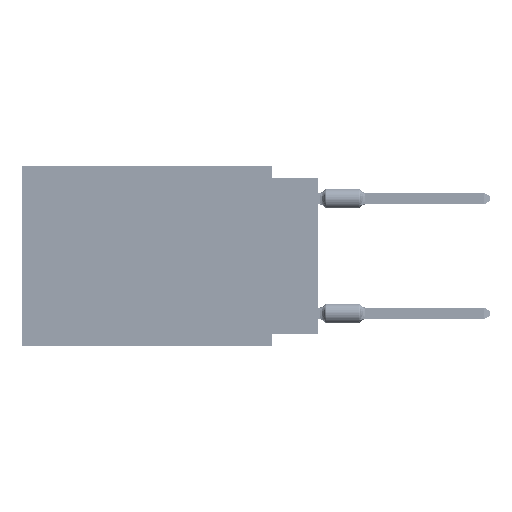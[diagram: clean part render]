
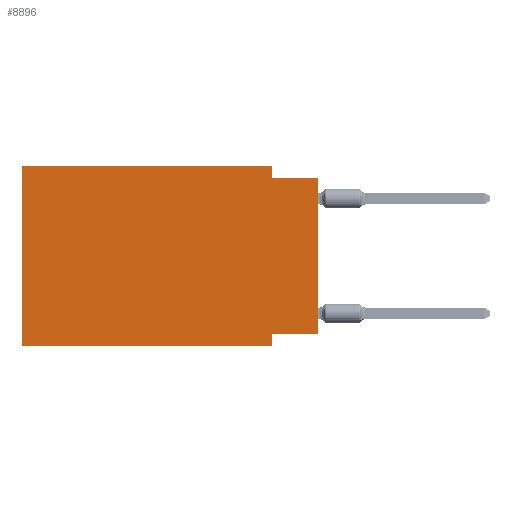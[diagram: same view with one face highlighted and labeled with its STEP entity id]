
A CAD part, left-side view. The second image highlights one B-rep face of the part: STEP entity #8896.
In plain terms, the highlighted planar face has unit normal (-1, 0, 0).
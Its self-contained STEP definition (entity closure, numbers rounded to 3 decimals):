
#1337 = DIRECTION ( 'NONE',  ( 0., -1., 0. ) ) ;
#1501 = DIRECTION ( 'NONE',  ( 0., 0., -1. ) ) ;
#1693 = LINE ( 'NONE', #13093, #30020 ) ;
#6231 = VECTOR ( 'NONE', #54330, 1000. ) ;
#6810 = CARTESIAN_POINT ( 'NONE',  ( 0., 2.54, -9.906 ) ) ;
#7722 = DIRECTION ( 'NONE',  ( 0., 0., -1. ) ) ;
#7745 = ORIENTED_EDGE ( 'NONE', *, *, #40765, .F. ) ;
#8896 = ADVANCED_FACE ( 'NONE', ( #43384 ), #11657, .F. ) ;
#9200 = CARTESIAN_POINT ( 'NONE',  ( 0., 0., -9.271 ) ) ;
#9477 = VECTOR ( 'NONE', #47346, 1000. ) ;
#9955 = DIRECTION ( 'NONE',  ( 0., 1., 0. ) ) ;
#11115 = EDGE_CURVE ( 'NONE', #29939, #39535, #31661, .T. ) ;
#11657 = PLANE ( 'NONE',  #27495 ) ;
#13093 = CARTESIAN_POINT ( 'NONE',  ( 0., 16.383, 0. ) ) ;
#13127 = EDGE_CURVE ( 'NONE', #60699, #47284, #43484, .T. ) ;
#15398 = CARTESIAN_POINT ( 'NONE',  ( 0., 0., -0.635 ) ) ;
#18947 = EDGE_CURVE ( 'NONE', #60699, #28085, #57865, .T. ) ;
#20659 = CARTESIAN_POINT ( 'NONE',  ( 0., 0., -9.271 ) ) ;
#22760 = VECTOR ( 'NONE', #9955, 1000. ) ;
#23958 = LINE ( 'NONE', #51034, #54979 ) ;
#24222 = VECTOR ( 'NONE', #29373, 1000. ) ;
#25728 = EDGE_LOOP ( 'NONE', ( #63925, #7745, #42499, #32569, #37279, #26729, #42286, #35473 ) ) ;
#26729 = ORIENTED_EDGE ( 'NONE', *, *, #18947, .T. ) ;
#26759 = CARTESIAN_POINT ( 'NONE',  ( 0., 2.54, -9.271 ) ) ;
#27492 = DIRECTION ( 'NONE',  ( 0., -1., 0. ) ) ;
#27495 = AXIS2_PLACEMENT_3D ( 'NONE', #61201, #44085, #7722 ) ;
#28085 = VERTEX_POINT ( 'NONE', #6810 ) ;
#29373 = DIRECTION ( 'NONE',  ( 0., -1., 0. ) ) ;
#29939 = VERTEX_POINT ( 'NONE', #9200 ) ;
#30020 = VECTOR ( 'NONE', #1337, 1000. ) ;
#31661 = LINE ( 'NONE', #53740, #9477 ) ;
#32569 = ORIENTED_EDGE ( 'NONE', *, *, #57169, .F. ) ;
#32605 = CARTESIAN_POINT ( 'NONE',  ( 0., 2.54, 0. ) ) ;
#32816 = DIRECTION ( 'NONE',  ( 0., 0., 1. ) ) ;
#35473 = ORIENTED_EDGE ( 'NONE', *, *, #41230, .F. ) ;
#36108 = LINE ( 'NONE', #15398, #43149 ) ;
#37279 = ORIENTED_EDGE ( 'NONE', *, *, #13127, .F. ) ;
#39314 = CARTESIAN_POINT ( 'NONE',  ( 0., 16.383, 0. ) ) ;
#39535 = VERTEX_POINT ( 'NONE', #57464 ) ;
#40765 = EDGE_CURVE ( 'NONE', #44817, #39535, #36108, .T. ) ;
#41230 = EDGE_CURVE ( 'NONE', #29939, #55328, #43427, .T. ) ;
#41494 = CARTESIAN_POINT ( 'NONE',  ( 0., 16.383, 0. ) ) ;
#42286 = ORIENTED_EDGE ( 'NONE', *, *, #61474, .F. ) ;
#42499 = ORIENTED_EDGE ( 'NONE', *, *, #45817, .F. ) ;
#43149 = VECTOR ( 'NONE', #27492, 1000. ) ;
#43384 = FACE_OUTER_BOUND ( 'NONE', #25728, .T. ) ;
#43427 = LINE ( 'NONE', #20659, #22760 ) ;
#43484 = LINE ( 'NONE', #41494, #46465 ) ;
#44085 = DIRECTION ( 'NONE',  ( 1., 0., 0. ) ) ;
#44817 = VERTEX_POINT ( 'NONE', #58439 ) ;
#45817 = EDGE_CURVE ( 'NONE', #63517, #44817, #59673, .T. ) ;
#46465 = VECTOR ( 'NONE', #32816, 1000. ) ;
#47284 = VERTEX_POINT ( 'NONE', #39314 ) ;
#47346 = DIRECTION ( 'NONE',  ( 0., 0., 1. ) ) ;
#47956 = CARTESIAN_POINT ( 'NONE',  ( 0., 16.383, -9.906 ) ) ;
#51034 = CARTESIAN_POINT ( 'NONE',  ( 0., 2.54, -9.906 ) ) ;
#53740 = CARTESIAN_POINT ( 'NONE',  ( 0., 0., 0. ) ) ;
#54330 = DIRECTION ( 'NONE',  ( 0., 0., -1. ) ) ;
#54979 = VECTOR ( 'NONE', #1501, 1000. ) ;
#55328 = VERTEX_POINT ( 'NONE', #26759 ) ;
#57169 = EDGE_CURVE ( 'NONE', #47284, #63517, #1693, .T. ) ;
#57464 = CARTESIAN_POINT ( 'NONE',  ( 0., 0., -0.635 ) ) ;
#57865 = LINE ( 'NONE', #63204, #24222 ) ;
#58439 = CARTESIAN_POINT ( 'NONE',  ( 0., 2.54, -0.635 ) ) ;
#59673 = LINE ( 'NONE', #32605, #6231 ) ;
#60699 = VERTEX_POINT ( 'NONE', #47956 ) ;
#61201 = CARTESIAN_POINT ( 'NONE',  ( 0., 16.383, 0. ) ) ;
#61474 = EDGE_CURVE ( 'NONE', #55328, #28085, #23958, .T. ) ;
#63204 = CARTESIAN_POINT ( 'NONE',  ( 0., 16.383, -9.906 ) ) ;
#63400 = CARTESIAN_POINT ( 'NONE',  ( 0., 2.54, 0. ) ) ;
#63517 = VERTEX_POINT ( 'NONE', #63400 ) ;
#63925 = ORIENTED_EDGE ( 'NONE', *, *, #11115, .T. ) ;
